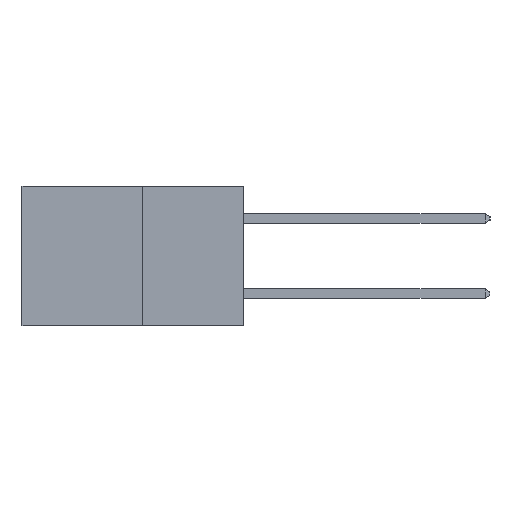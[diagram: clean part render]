
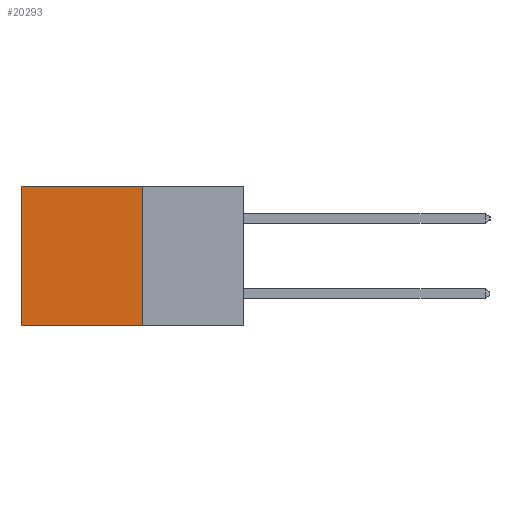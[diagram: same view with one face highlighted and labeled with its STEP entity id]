
A CAD part, left-side view. The second image highlights one B-rep face of the part: STEP entity #20293.
In plain terms, the highlighted planar face has unit normal (-1, 0, 0).
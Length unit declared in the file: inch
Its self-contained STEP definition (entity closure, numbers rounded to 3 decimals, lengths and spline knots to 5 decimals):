
#448 = LINE ( 'NONE', #6167, #17147 ) ;
#483 = ORIENTED_EDGE ( 'NONE', *, *, #10150, .T. ) ;
#504 = ORIENTED_EDGE ( 'NONE', *, *, #6207, .F. ) ;
#1165 = VERTEX_POINT ( 'NONE', #15447 ) ;
#2050 = VERTEX_POINT ( 'NONE', #2387 ) ;
#2387 = CARTESIAN_POINT ( 'NONE',  ( 0.277, 0.59, 0. ) ) ;
#2471 = CARTESIAN_POINT ( 'NONE',  ( 0.277, 0.27, -0.37 ) ) ;
#2994 = DIRECTION ( 'NONE',  ( 0., 0., -1. ) ) ;
#4950 = CARTESIAN_POINT ( 'NONE',  ( 0.277, 0.27, 0. ) ) ;
#5288 = VECTOR ( 'NONE', #2994, 39.37008 ) ;
#6167 = CARTESIAN_POINT ( 'NONE',  ( 0.277, 0.27, 0. ) ) ;
#6207 = EDGE_CURVE ( 'NONE', #17576, #10436, #9636, .T. ) ;
#6656 = CARTESIAN_POINT ( 'NONE',  ( 0.277, 0.27, -0.37 ) ) ;
#7271 = VECTOR ( 'NONE', #14686, 39.37008 ) ;
#7820 = DIRECTION ( 'NONE',  ( 0., 1., 0. ) ) ;
#7939 = CARTESIAN_POINT ( 'NONE',  ( 0.277, 0.27, -0.37 ) ) ;
#9573 = DIRECTION ( 'NONE',  ( 0., 0., -1. ) ) ;
#9636 = LINE ( 'NONE', #2471, #5288 ) ;
#10150 = EDGE_CURVE ( 'NONE', #17576, #2050, #448, .T. ) ;
#10436 = VERTEX_POINT ( 'NONE', #13382 ) ;
#10543 = AXIS2_PLACEMENT_3D ( 'NONE', #7939, #19007, #9573 ) ;
#10860 = EDGE_LOOP ( 'NONE', ( #16817, #13207, #504, #483 ) ) ;
#12484 = FACE_OUTER_BOUND ( 'NONE', #10860, .T. ) ;
#12495 = DIRECTION ( 'NONE',  ( 0., 0., -1. ) ) ;
#13207 = ORIENTED_EDGE ( 'NONE', *, *, #18282, .F. ) ;
#13382 = CARTESIAN_POINT ( 'NONE',  ( 0.277, 0.27, -0.37 ) ) ;
#14686 = DIRECTION ( 'NONE',  ( 0., 1., 0. ) ) ;
#15447 = CARTESIAN_POINT ( 'NONE',  ( 0.277, 0.59, -0.37 ) ) ;
#16254 = LINE ( 'NONE', #6656, #7271 ) ;
#16507 = LINE ( 'NONE', #20209, #20099 ) ;
#16817 = ORIENTED_EDGE ( 'NONE', *, *, #18011, .T. ) ;
#17147 = VECTOR ( 'NONE', #7820, 39.37008 ) ;
#17449 = PLANE ( 'NONE',  #10543 ) ;
#17576 = VERTEX_POINT ( 'NONE', #4950 ) ;
#18011 = EDGE_CURVE ( 'NONE', #2050, #1165, #16507, .T. ) ;
#18282 = EDGE_CURVE ( 'NONE', #10436, #1165, #16254, .T. ) ;
#19007 = DIRECTION ( 'NONE',  ( 1., 0., 0. ) ) ;
#20099 = VECTOR ( 'NONE', #12495, 39.37008 ) ;
#20209 = CARTESIAN_POINT ( 'NONE',  ( 0.277, 0.59, -0.37 ) ) ;
#20293 = ADVANCED_FACE ( 'NONE', ( #12484 ), #17449, .F. ) ;
